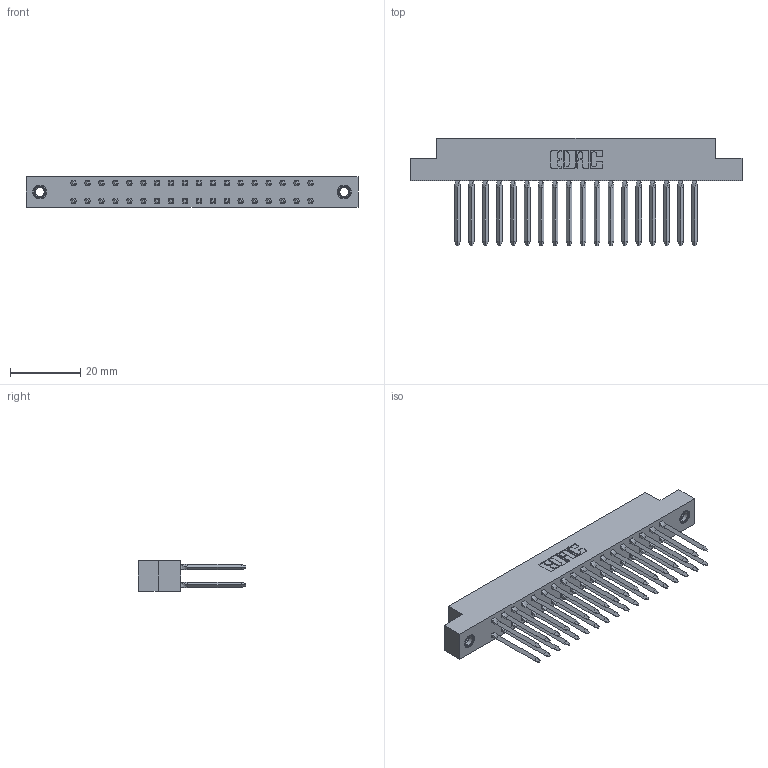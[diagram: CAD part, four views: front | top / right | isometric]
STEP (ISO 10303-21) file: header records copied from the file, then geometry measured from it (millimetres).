
FILE_DESCRIPTION (( 'STEP AP203' ), '1' );
FILE_NAME ('338-036-541-207.STEP', '2020-03-24T18:27:32', ( '' ), ( '' ), 'SwSTEP 2.0', 'SolidWorks 2016', '' );
FILE_SCHEMA (( 'CONFIG_CONTROL_DESIGN' ));
Length unit declared in the file: inch
Products named in the file (4): 345-250-001_345-250-005-103; 338-210-001_338-210-018-004; 338-290-001_541; 338-036-541-207
Assembly tree (39 placements, depth 2):
  338-036-541-207
    338-210-001_338-210-018-004
    338-290-001_541  x36
    345-250-001_345-250-005-103  x2
Bounding box: 94.34 x 30.56 x 8.71 mm (x, y, z)
Volume: 7187.9 mm3; surface area: 13095.5 mm2
Topology: 39 solids, 39 shells, 2566 faces, 6867 edges, 4354 vertices
Faces by surface type: plane 1774, cylinder 632, bspline 144, cone 12, torus 4
Entity records: 38813 total; most frequent: CARTESIAN_POINT 7683, ORIENTED_EDGE 6424, DIRECTION 6041, EDGE_CURVE 3212, LINE 2373, VECTOR 2373, VERTEX_POINT 2084, AXIS2_PLACEMENT_3D 1834
